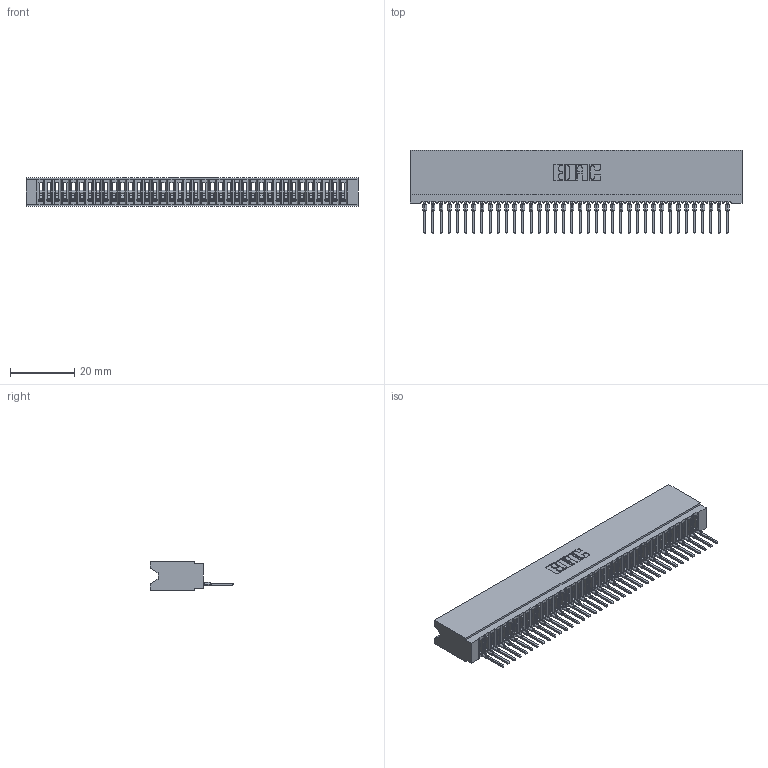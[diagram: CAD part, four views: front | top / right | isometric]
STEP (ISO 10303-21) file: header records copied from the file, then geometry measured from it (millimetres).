
FILE_DESCRIPTION (( 'STEP AP203' ), '1' );
FILE_NAME ('745-038-522-106.STEP', '2026-02-25T18:47:05', ( '' ), ( '' ), 'SwSTEP 2.0', 'SolidWorks 2023', '' );
FILE_SCHEMA (( 'CONFIG_CONTROL_DESIGN' ));
Length unit declared in the file: millimetre
Products named in the file (3): 745-038-522-106; 745 Part_Insulator Option - 06; 745-292-001_522
Assembly tree (39 placements, depth 2):
  745-038-522-106
    745 Part_Insulator Option - 06
    745-292-001_522  x38
Bounding box: 103.12 x 25.92 x 8.89 mm (x, y, z)
Volume: 8956.7 mm3; surface area: 16731.4 mm2
Topology: 39 solids, 39 shells, 4352 faces, 11964 edges, 7544 vertices
Faces by surface type: plane 2602, cylinder 762, bspline 760, torus 228
Entity records: 63324 total; most frequent: CARTESIAN_POINT 11660, ORIENTED_EDGE 11126, DIRECTION 9647, EDGE_CURVE 5563, VECTOR 5153, LINE 5153, VERTEX_POINT 3548, AXIS2_PLACEMENT_3D 2247
